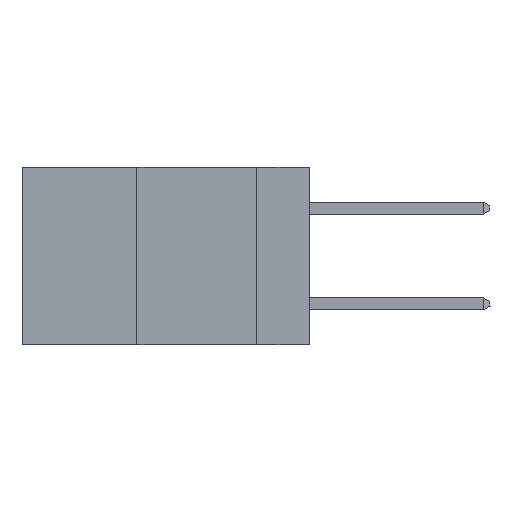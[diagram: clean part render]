
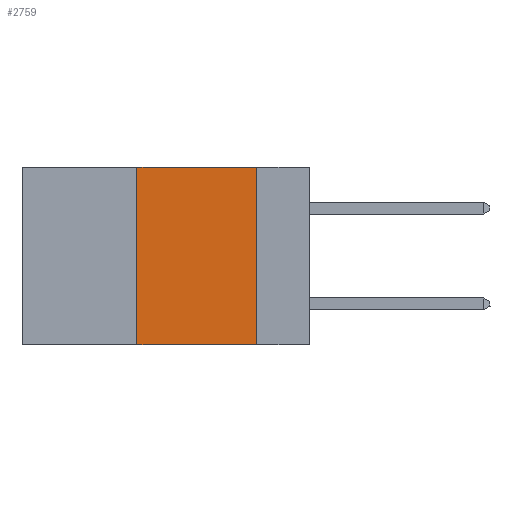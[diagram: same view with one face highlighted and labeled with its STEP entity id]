
A CAD part, left-side view. The second image highlights one B-rep face of the part: STEP entity #2759.
In plain terms, the highlighted planar face has unit normal (-1, 0, 0).
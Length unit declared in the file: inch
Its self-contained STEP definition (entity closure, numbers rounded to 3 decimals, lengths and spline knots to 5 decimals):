
#2029 = DIRECTION ( 'NONE',  ( 0., -1., 0. ) ) ;
#2542 = ORIENTED_EDGE ( 'NONE', *, *, #3902, .F. ) ;
#2759 = ADVANCED_FACE ( 'NONE', ( #3310 ), #13110, .F. ) ;
#3310 = FACE_OUTER_BOUND ( 'NONE', #4165, .T. ) ;
#3902 = EDGE_CURVE ( 'NONE', #27307, #14968, #9854, .T. ) ;
#3958 = EDGE_CURVE ( 'NONE', #14968, #23644, #22433, .T. ) ;
#4165 = EDGE_LOOP ( 'NONE', ( #26012, #2542, #23735, #29504 ) ) ;
#5437 = CARTESIAN_POINT ( 'NONE',  ( 0., 0.6, 0. ) ) ;
#6938 = LINE ( 'NONE', #31589, #20557 ) ;
#8241 = CARTESIAN_POINT ( 'NONE',  ( 0., 0.36, -0.37 ) ) ;
#9272 = LINE ( 'NONE', #11564, #29389 ) ;
#9829 = CARTESIAN_POINT ( 'NONE',  ( 0., 0.36, 0. ) ) ;
#9854 = LINE ( 'NONE', #26997, #24978 ) ;
#11564 = CARTESIAN_POINT ( 'NONE',  ( 0., 0.36, 0. ) ) ;
#13110 = PLANE ( 'NONE',  #16424 ) ;
#14927 = CARTESIAN_POINT ( 'NONE',  ( 0., 0.11, -0.37 ) ) ;
#14968 = VERTEX_POINT ( 'NONE', #17953 ) ;
#15408 = DIRECTION ( 'NONE',  ( 1., 0., 0. ) ) ;
#15733 = DIRECTION ( 'NONE',  ( 0., 0., -1. ) ) ;
#16424 = AXIS2_PLACEMENT_3D ( 'NONE', #5437, #15408, #15733 ) ;
#17240 = DIRECTION ( 'NONE',  ( 0., 0., -1. ) ) ;
#17953 = CARTESIAN_POINT ( 'NONE',  ( 0., 0.11, 0. ) ) ;
#19999 = VERTEX_POINT ( 'NONE', #8241 ) ;
#20557 = VECTOR ( 'NONE', #2029, 39.37008 ) ;
#22433 = LINE ( 'NONE', #27634, #28126 ) ;
#23644 = VERTEX_POINT ( 'NONE', #14927 ) ;
#23735 = ORIENTED_EDGE ( 'NONE', *, *, #24397, .F. ) ;
#24397 = EDGE_CURVE ( 'NONE', #19999, #27307, #9272, .T. ) ;
#24758 = EDGE_CURVE ( 'NONE', #19999, #23644, #6938, .T. ) ;
#24978 = VECTOR ( 'NONE', #29460, 39.37008 ) ;
#26012 = ORIENTED_EDGE ( 'NONE', *, *, #3958, .F. ) ;
#26997 = CARTESIAN_POINT ( 'NONE',  ( 0., 0.6, 0. ) ) ;
#27307 = VERTEX_POINT ( 'NONE', #9829 ) ;
#27634 = CARTESIAN_POINT ( 'NONE',  ( 0., 0.11, 0. ) ) ;
#28126 = VECTOR ( 'NONE', #17240, 39.37008 ) ;
#29389 = VECTOR ( 'NONE', #31460, 39.37008 ) ;
#29460 = DIRECTION ( 'NONE',  ( 0., -1., 0. ) ) ;
#29504 = ORIENTED_EDGE ( 'NONE', *, *, #24758, .T. ) ;
#31460 = DIRECTION ( 'NONE',  ( 0., 0., 1. ) ) ;
#31589 = CARTESIAN_POINT ( 'NONE',  ( 0., 0.6, -0.37 ) ) ;
